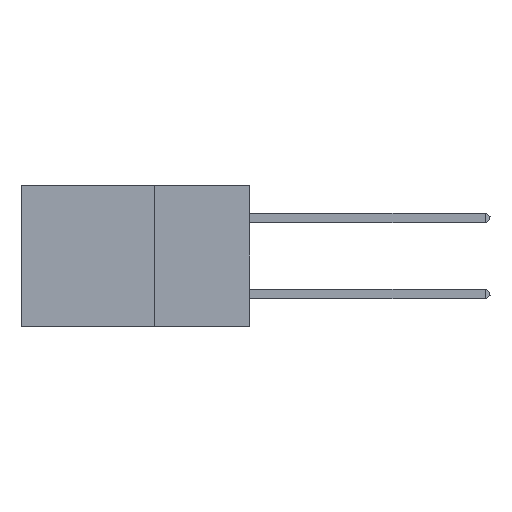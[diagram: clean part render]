
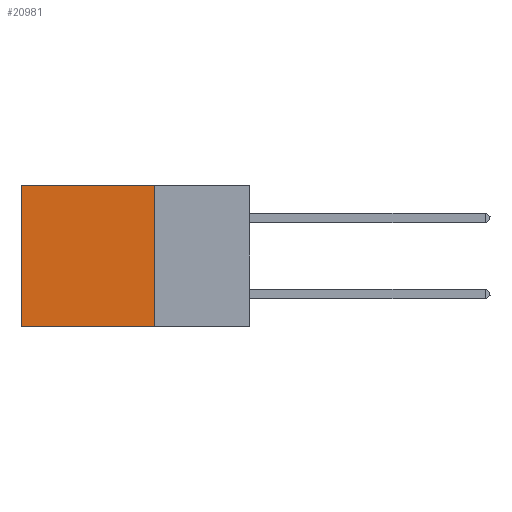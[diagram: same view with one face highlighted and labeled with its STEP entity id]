
A CAD part, left-side view. The second image highlights one B-rep face of the part: STEP entity #20981.
In plain terms, the highlighted planar face has unit normal (-1, 0, 0).
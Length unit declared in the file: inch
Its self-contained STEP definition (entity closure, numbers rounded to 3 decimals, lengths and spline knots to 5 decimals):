
#760 = VERTEX_POINT ( 'NONE', #29254 ) ;
#1240 = DIRECTION ( 'NONE',  ( 0., 0., -1. ) ) ;
#2106 = CARTESIAN_POINT ( 'NONE',  ( 0.2875, 0.25, -0.37 ) ) ;
#2227 = DIRECTION ( 'NONE',  ( 0., 0., -1. ) ) ;
#4294 = ORIENTED_EDGE ( 'NONE', *, *, #13259, .T. ) ;
#4385 = LINE ( 'NONE', #42213, #43190 ) ;
#4915 = VERTEX_POINT ( 'NONE', #16447 ) ;
#5010 = VERTEX_POINT ( 'NONE', #23483 ) ;
#5134 = CARTESIAN_POINT ( 'NONE',  ( 0.2875, 0.25, 0. ) ) ;
#5522 = VECTOR ( 'NONE', #1240, 39.37008 ) ;
#6344 = LINE ( 'NONE', #7603, #32540 ) ;
#7603 = CARTESIAN_POINT ( 'NONE',  ( 0.2875, 0.25, 0. ) ) ;
#9081 = DIRECTION ( 'NONE',  ( 1., 0., 0. ) ) ;
#10962 = DIRECTION ( 'NONE',  ( 0., 1., 0. ) ) ;
#12605 = DIRECTION ( 'NONE',  ( 0., 0., -1. ) ) ;
#13259 = EDGE_CURVE ( 'NONE', #4915, #5010, #38517, .T. ) ;
#14019 = LINE ( 'NONE', #2106, #35507 ) ;
#16292 = ORIENTED_EDGE ( 'NONE', *, *, #30238, .F. ) ;
#16447 = CARTESIAN_POINT ( 'NONE',  ( 0.2875, 0.6, 0. ) ) ;
#19329 = CARTESIAN_POINT ( 'NONE',  ( 0.2875, 0.25, 0. ) ) ;
#19688 = ORIENTED_EDGE ( 'NONE', *, *, #32354, .F. ) ;
#20981 = ADVANCED_FACE ( 'NONE', ( #23669 ), #42461, .F. ) ;
#23483 = CARTESIAN_POINT ( 'NONE',  ( 0.2875, 0.6, -0.37 ) ) ;
#23669 = FACE_OUTER_BOUND ( 'NONE', #41367, .T. ) ;
#27873 = CARTESIAN_POINT ( 'NONE',  ( 0.2875, 0.6, 0. ) ) ;
#29254 = CARTESIAN_POINT ( 'NONE',  ( 0.2875, 0.25, -0.37 ) ) ;
#30238 = EDGE_CURVE ( 'NONE', #760, #5010, #14019, .T. ) ;
#31631 = AXIS2_PLACEMENT_3D ( 'NONE', #19329, #9081, #12605 ) ;
#32354 = EDGE_CURVE ( 'NONE', #40258, #760, #4385, .T. ) ;
#32540 = VECTOR ( 'NONE', #10962, 39.37008 ) ;
#35460 = DIRECTION ( 'NONE',  ( 0., 1., 0. ) ) ;
#35507 = VECTOR ( 'NONE', #35460, 39.37008 ) ;
#36901 = EDGE_CURVE ( 'NONE', #40258, #4915, #6344, .T. ) ;
#38517 = LINE ( 'NONE', #27873, #5522 ) ;
#40258 = VERTEX_POINT ( 'NONE', #5134 ) ;
#41367 = EDGE_LOOP ( 'NONE', ( #4294, #16292, #19688, #41609 ) ) ;
#41609 = ORIENTED_EDGE ( 'NONE', *, *, #36901, .T. ) ;
#42213 = CARTESIAN_POINT ( 'NONE',  ( 0.2875, 0.25, 0. ) ) ;
#42461 = PLANE ( 'NONE',  #31631 ) ;
#43190 = VECTOR ( 'NONE', #2227, 39.37008 ) ;
